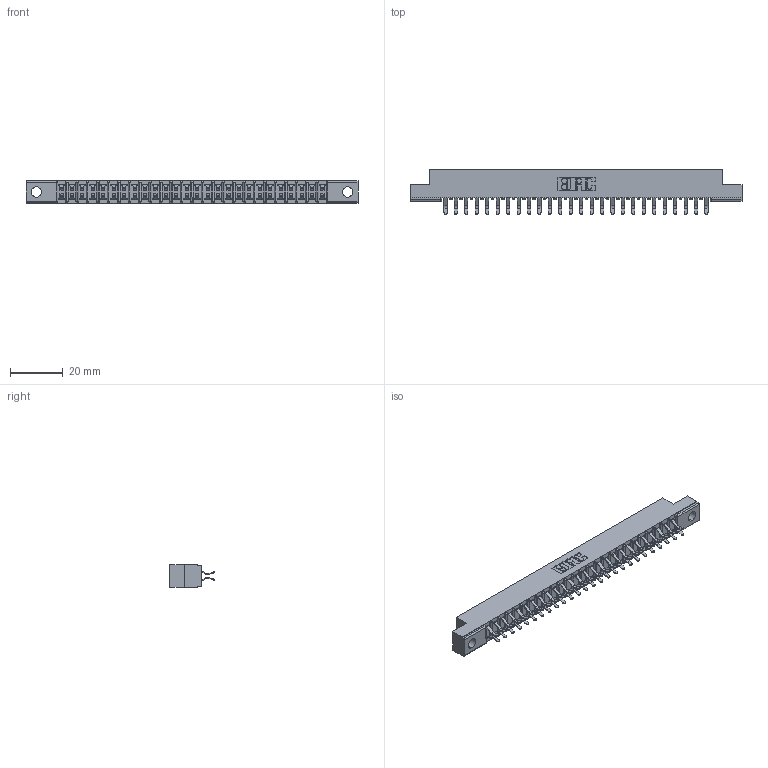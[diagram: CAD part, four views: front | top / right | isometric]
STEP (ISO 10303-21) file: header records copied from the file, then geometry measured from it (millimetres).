
FILE_DESCRIPTION (( 'STEP AP203' ), '1' );
FILE_NAME ('357-052-556-204.STEP', '2019-09-19T03:31:55', ( '' ), ( '' ), 'SwSTEP 2.0', 'SolidWorks 2016', '' );
FILE_SCHEMA (( 'CONFIG_CONTROL_DESIGN' ));
Length unit declared in the file: inch
Products named in the file (3): 357-052-556-204; 307 Part_.156 Dia Mounting Holes; 307-290-001_556
Assembly tree (53 placements, depth 2):
  357-052-556-204
    307 Part_.156 Dia Mounting Holes
    307-290-001_556  x52
Bounding box: 126.03 x 16.97 x 8.71 mm (x, y, z)
Volume: 8128.2 mm3; surface area: 14401.4 mm2
Topology: 53 solids, 53 shells, 2759 faces, 7743 edges, 5018 vertices
Faces by surface type: plane 1800, cylinder 905, sphere 54
Entity records: 25616 total; most frequent: CARTESIAN_POINT 4200, ORIENTED_EDGE 4158, DIRECTION 4113, EDGE_CURVE 2079, LINE 1595, VECTOR 1595, VERTEX_POINT 1346, AXIS2_PLACEMENT_3D 1259
